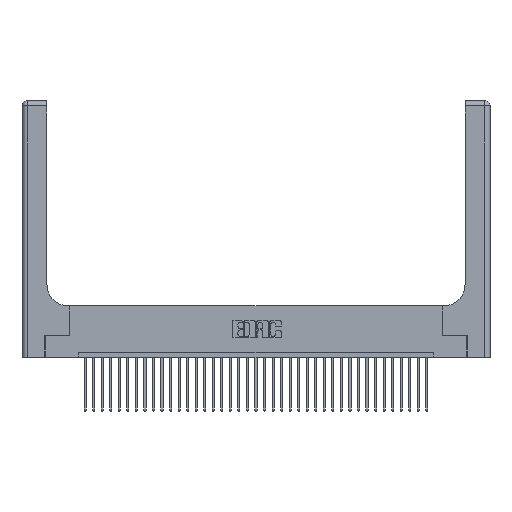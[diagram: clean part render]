
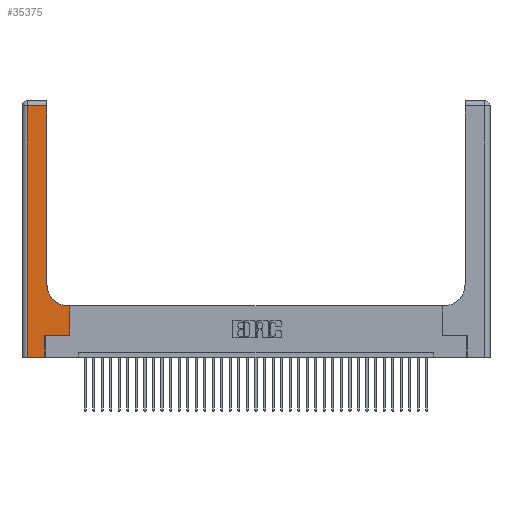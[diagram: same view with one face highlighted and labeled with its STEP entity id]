
A CAD part, top view. The second image highlights one B-rep face of the part: STEP entity #35375.
In plain terms, the highlighted planar face has unit normal (0, 0, 1).
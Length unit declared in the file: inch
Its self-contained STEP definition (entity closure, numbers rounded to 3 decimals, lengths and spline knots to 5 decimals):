
#987 = ORIENTED_EDGE ( 'NONE', *, *, #4964, .T. ) ;
#1979 = PLANE ( 'NONE',  #35343 ) ;
#2935 = EDGE_CURVE ( 'NONE', #33590, #33634, #24153, .T. ) ;
#3692 = DIRECTION ( 'NONE',  ( -1., 0., 0. ) ) ;
#4400 = ORIENTED_EDGE ( 'NONE', *, *, #33048, .T. ) ;
#4531 = CARTESIAN_POINT ( 'NONE',  ( 0.2915, 0.85, 0.37 ) ) ;
#4780 = CARTESIAN_POINT ( 'NONE',  ( 0., 3., 0.37 ) ) ;
#4964 = EDGE_CURVE ( 'NONE', #5062, #8056, #9166, .T. ) ;
#5062 = VERTEX_POINT ( 'NONE', #16637 ) ;
#5263 = CARTESIAN_POINT ( 'NONE',  ( 0.06, 2.94, 0.37 ) ) ;
#5545 = ORIENTED_EDGE ( 'NONE', *, *, #20700, .T. ) ;
#5636 = LINE ( 'NONE', #11806, #20082 ) ;
#6406 = LINE ( 'NONE', #30353, #17758 ) ;
#6625 = DIRECTION ( 'NONE',  ( 0., 0., -1. ) ) ;
#6845 = EDGE_CURVE ( 'NONE', #30917, #29067, #17770, .T. ) ;
#7958 = DIRECTION ( 'NONE',  ( 0., 1., 0. ) ) ;
#7970 = ORIENTED_EDGE ( 'NONE', *, *, #2935, .T. ) ;
#8050 = CARTESIAN_POINT ( 'NONE',  ( 0.2915, 3., 0.37 ) ) ;
#8056 = VERTEX_POINT ( 'NONE', #9974 ) ;
#8333 = AXIS2_PLACEMENT_3D ( 'NONE', #12226, #6625, #21033 ) ;
#8887 = ORIENTED_EDGE ( 'NONE', *, *, #30991, .T. ) ;
#8975 = LINE ( 'NONE', #12844, #32564 ) ;
#9166 = LINE ( 'NONE', #19089, #29734 ) ;
#9447 = VECTOR ( 'NONE', #31146, 39.37008 ) ;
#9974 = CARTESIAN_POINT ( 'NONE',  ( 0.5585, 0.6, 0.37 ) ) ;
#10596 = FACE_OUTER_BOUND ( 'NONE', #32477, .T. ) ;
#10631 = CARTESIAN_POINT ( 'NONE',  ( 0.06, 0., 0.37 ) ) ;
#10639 = DIRECTION ( 'NONE',  ( 0., 0., -1. ) ) ;
#11288 = VERTEX_POINT ( 'NONE', #4531 ) ;
#11437 = CARTESIAN_POINT ( 'NONE',  ( 0.269, 0., 0.37 ) ) ;
#11806 = CARTESIAN_POINT ( 'NONE',  ( 0., 2.94, 0.37 ) ) ;
#12013 = EDGE_CURVE ( 'NONE', #32743, #33590, #5636, .T. ) ;
#12226 = CARTESIAN_POINT ( 'NONE',  ( 0.5415, 0.85, 0.37 ) ) ;
#12844 = CARTESIAN_POINT ( 'NONE',  ( 0., 0., 0.37 ) ) ;
#13494 = EDGE_CURVE ( 'NONE', #29067, #5062, #6406, .T. ) ;
#13854 = CARTESIAN_POINT ( 'NONE',  ( 0.06, 3., 0.37 ) ) ;
#13926 = CIRCLE ( 'NONE', #8333, 0.25 ) ;
#13954 = DIRECTION ( 'NONE',  ( 1., 0., 0. ) ) ;
#15063 = LINE ( 'NONE', #8050, #17285 ) ;
#15334 = ORIENTED_EDGE ( 'NONE', *, *, #12013, .T. ) ;
#15849 = ORIENTED_EDGE ( 'NONE', *, *, #26943, .T. ) ;
#16637 = CARTESIAN_POINT ( 'NONE',  ( 0.5585, 0.25, 0.37 ) ) ;
#17285 = VECTOR ( 'NONE', #32737, 39.37008 ) ;
#17758 = VECTOR ( 'NONE', #13954, 39.37008 ) ;
#17770 = LINE ( 'NONE', #11437, #9447 ) ;
#18428 = ORIENTED_EDGE ( 'NONE', *, *, #13494, .T. ) ;
#19089 = CARTESIAN_POINT ( 'NONE',  ( 0.5585, 0.25, 0.37 ) ) ;
#19602 = DIRECTION ( 'NONE',  ( 0., -1., 0. ) ) ;
#20082 = VECTOR ( 'NONE', #31735, 39.37008 ) ;
#20565 = CARTESIAN_POINT ( 'NONE',  ( 0.2915, 0.6, 0.37 ) ) ;
#20700 = EDGE_CURVE ( 'NONE', #33634, #30917, #8975, .T. ) ;
#21033 = DIRECTION ( 'NONE',  ( 1., 0., 0. ) ) ;
#24153 = LINE ( 'NONE', #13854, #28953 ) ;
#24337 = DIRECTION ( 'NONE',  ( -1., 0., 0. ) ) ;
#25943 = CARTESIAN_POINT ( 'NONE',  ( 0.2915, 2.94, 0.37 ) ) ;
#26392 = VECTOR ( 'NONE', #3692, 39.37008 ) ;
#26674 = DIRECTION ( 'NONE',  ( 1., 0., 0. ) ) ;
#26943 = EDGE_CURVE ( 'NONE', #8056, #30327, #27686, .T. ) ;
#27686 = LINE ( 'NONE', #20565, #26392 ) ;
#28816 = CARTESIAN_POINT ( 'NONE',  ( 0.269, 0.25, 0.37 ) ) ;
#28953 = VECTOR ( 'NONE', #19602, 39.37008 ) ;
#29067 = VERTEX_POINT ( 'NONE', #28816 ) ;
#29708 = CARTESIAN_POINT ( 'NONE',  ( 0.5415, 0.6, 0.37 ) ) ;
#29734 = VECTOR ( 'NONE', #7958, 39.37008 ) ;
#30327 = VERTEX_POINT ( 'NONE', #29708 ) ;
#30353 = CARTESIAN_POINT ( 'NONE',  ( 0.269, 0.25, 0.37 ) ) ;
#30917 = VERTEX_POINT ( 'NONE', #34590 ) ;
#30991 = EDGE_CURVE ( 'NONE', #30327, #11288, #13926, .T. ) ;
#31146 = DIRECTION ( 'NONE',  ( 0., 1., 0. ) ) ;
#31735 = DIRECTION ( 'NONE',  ( -1., 0., 0. ) ) ;
#32477 = EDGE_LOOP ( 'NONE', ( #4400, #15334, #7970, #5545, #33577, #18428, #987, #15849, #8887 ) ) ;
#32564 = VECTOR ( 'NONE', #26674, 39.37008 ) ;
#32737 = DIRECTION ( 'NONE',  ( 0., 1., 0. ) ) ;
#32743 = VERTEX_POINT ( 'NONE', #25943 ) ;
#33048 = EDGE_CURVE ( 'NONE', #11288, #32743, #15063, .T. ) ;
#33577 = ORIENTED_EDGE ( 'NONE', *, *, #6845, .T. ) ;
#33590 = VERTEX_POINT ( 'NONE', #5263 ) ;
#33634 = VERTEX_POINT ( 'NONE', #10631 ) ;
#34590 = CARTESIAN_POINT ( 'NONE',  ( 0.269, 0., 0.37 ) ) ;
#35343 = AXIS2_PLACEMENT_3D ( 'NONE', #4780, #10639, #24337 ) ;
#35375 = ADVANCED_FACE ( 'NONE', ( #10596 ), #1979, .F. ) ;
